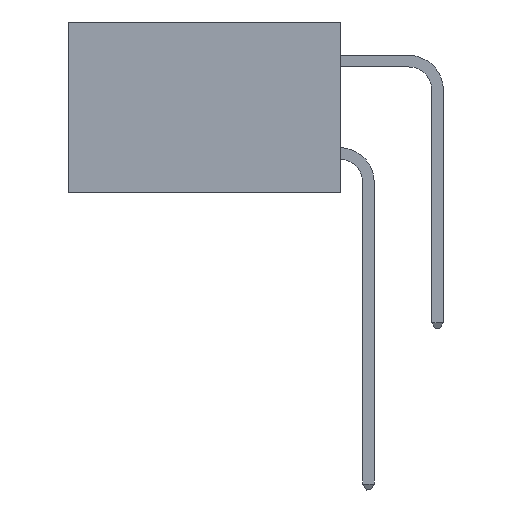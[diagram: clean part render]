
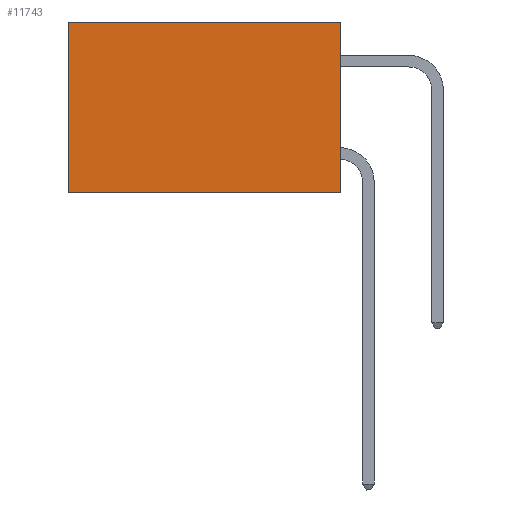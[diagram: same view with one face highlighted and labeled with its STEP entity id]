
A CAD part, left-side view. The second image highlights one B-rep face of the part: STEP entity #11743.
In plain terms, the highlighted planar face has unit normal (-1, 0, 0).
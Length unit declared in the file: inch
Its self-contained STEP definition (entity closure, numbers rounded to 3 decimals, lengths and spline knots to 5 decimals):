
#747 = EDGE_LOOP ( 'NONE', ( #4108, #5150, #14336, #20245 ) ) ;
#1858 = CARTESIAN_POINT ( 'NONE',  ( 0.277, 0., -0.37 ) ) ;
#2615 = LINE ( 'NONE', #14469, #11284 ) ;
#2989 = LINE ( 'NONE', #20237, #7327 ) ;
#3598 = EDGE_CURVE ( 'NONE', #20422, #15001, #12660, .T. ) ;
#3649 = CARTESIAN_POINT ( 'NONE',  ( 0.277, 0.59, 0. ) ) ;
#4108 = ORIENTED_EDGE ( 'NONE', *, *, #15131, .T. ) ;
#4279 = AXIS2_PLACEMENT_3D ( 'NONE', #4543, #20917, #11137 ) ;
#4543 = CARTESIAN_POINT ( 'NONE',  ( 0.277, 0., -0.37 ) ) ;
#4685 = DIRECTION ( 'NONE',  ( 0., 1., 0. ) ) ;
#5150 = ORIENTED_EDGE ( 'NONE', *, *, #11791, .F. ) ;
#7327 = VECTOR ( 'NONE', #10459, 39.37008 ) ;
#7401 = DIRECTION ( 'NONE',  ( 0., 0., -1. ) ) ;
#7419 = VECTOR ( 'NONE', #7401, 39.37008 ) ;
#7797 = VECTOR ( 'NONE', #16779, 39.37008 ) ;
#8478 = FACE_OUTER_BOUND ( 'NONE', #747, .T. ) ;
#9318 = VERTEX_POINT ( 'NONE', #1858 ) ;
#9657 = CARTESIAN_POINT ( 'NONE',  ( 0.277, 0., 0. ) ) ;
#10459 = DIRECTION ( 'NONE',  ( 0., 0., -1. ) ) ;
#11137 = DIRECTION ( 'NONE',  ( 0., 0., -1. ) ) ;
#11284 = VECTOR ( 'NONE', #4685, 39.37008 ) ;
#11743 = ADVANCED_FACE ( 'NONE', ( #8478 ), #14328, .F. ) ;
#11791 = EDGE_CURVE ( 'NONE', #9318, #20751, #2615, .T. ) ;
#12255 = EDGE_CURVE ( 'NONE', #20422, #9318, #15067, .T. ) ;
#12660 = LINE ( 'NONE', #18375, #7797 ) ;
#14328 = PLANE ( 'NONE',  #4279 ) ;
#14336 = ORIENTED_EDGE ( 'NONE', *, *, #12255, .F. ) ;
#14469 = CARTESIAN_POINT ( 'NONE',  ( 0.277, 0., -0.37 ) ) ;
#15001 = VERTEX_POINT ( 'NONE', #3649 ) ;
#15067 = LINE ( 'NONE', #17176, #7419 ) ;
#15131 = EDGE_CURVE ( 'NONE', #15001, #20751, #2989, .T. ) ;
#16779 = DIRECTION ( 'NONE',  ( 0., 1., 0. ) ) ;
#16903 = CARTESIAN_POINT ( 'NONE',  ( 0.277, 0.59, -0.37 ) ) ;
#17176 = CARTESIAN_POINT ( 'NONE',  ( 0.277, 0., -0.37 ) ) ;
#18375 = CARTESIAN_POINT ( 'NONE',  ( 0.277, 0., 0. ) ) ;
#20237 = CARTESIAN_POINT ( 'NONE',  ( 0.277, 0.59, -0.37 ) ) ;
#20245 = ORIENTED_EDGE ( 'NONE', *, *, #3598, .T. ) ;
#20422 = VERTEX_POINT ( 'NONE', #9657 ) ;
#20751 = VERTEX_POINT ( 'NONE', #16903 ) ;
#20917 = DIRECTION ( 'NONE',  ( 1., 0., 0. ) ) ;
